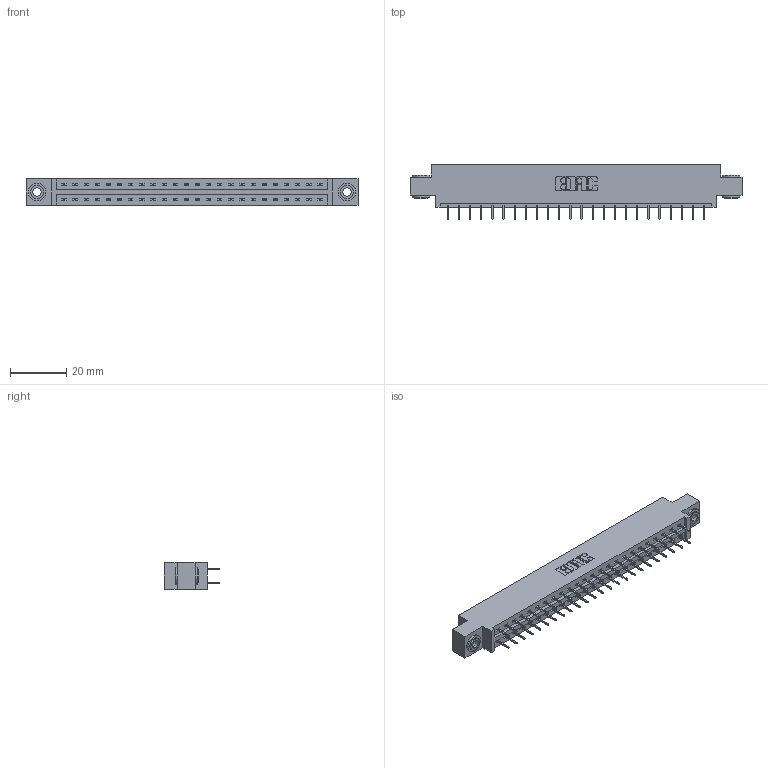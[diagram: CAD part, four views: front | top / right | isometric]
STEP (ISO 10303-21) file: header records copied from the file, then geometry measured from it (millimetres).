
FILE_DESCRIPTION (( 'STEP AP203' ), '1' );
FILE_NAME ('387-048-524-803.STEP', '2019-10-18T09:31:10', ( '' ), ( '' ), 'SwSTEP 2.0', 'SolidWorks 2016', '' );
FILE_SCHEMA (( 'CONFIG_CONTROL_DESIGN' ));
Length unit declared in the file: inch
Products named in the file (4): 337 Part_0.170 Offset - 0.156 Dia-TH; 387-048-524-803; 345-292-001_345-293-124; 345-250-002_345-250-002-102
Assembly tree (51 placements, depth 2):
  387-048-524-803
    337 Part_0.170 Offset - 0.156 Dia-TH
    345-292-001_345-293-124  x48
    345-250-002_345-250-002-102  x2
Bounding box: 118.11 x 19.69 x 9.4 mm (x, y, z)
Volume: 12037 mm3; surface area: 13540.3 mm2
Topology: 51 solids, 51 shells, 2940 faces, 8319 edges, 5350 vertices
Faces by surface type: plane 2196, cylinder 736, cone 8
Entity records: 21792 total; most frequent: CARTESIAN_POINT 3661, ORIENTED_EDGE 3590, DIRECTION 3181, EDGE_CURVE 1795, LINE 1647, VECTOR 1647, VERTEX_POINT 1190, AXIS2_PLACEMENT_3D 767
